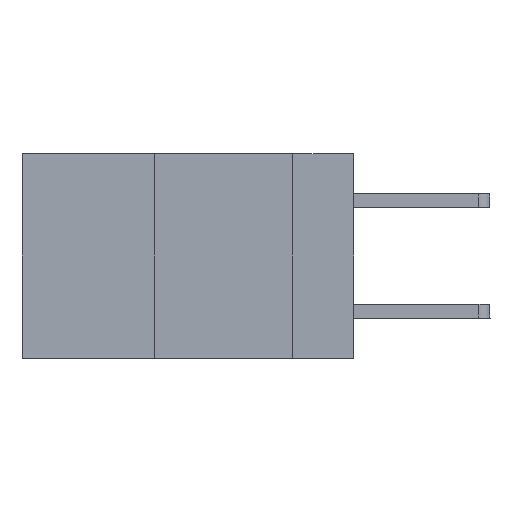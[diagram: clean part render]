
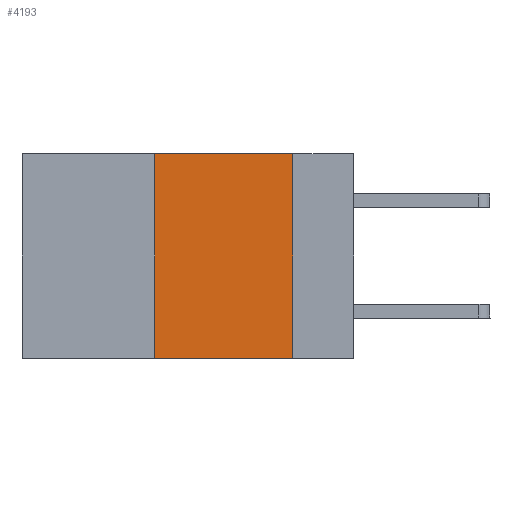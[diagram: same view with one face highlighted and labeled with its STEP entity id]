
A CAD part, left-side view. The second image highlights one B-rep face of the part: STEP entity #4193.
In plain terms, the highlighted planar face has unit normal (-1, 0, 0).
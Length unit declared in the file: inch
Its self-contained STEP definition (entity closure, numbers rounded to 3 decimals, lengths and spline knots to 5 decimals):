
#236 = DIRECTION ( 'NONE',  ( 1., 0., 0. ) ) ;
#2306 = ORIENTED_EDGE ( 'NONE', *, *, #3130, .F. ) ;
#2443 = ORIENTED_EDGE ( 'NONE', *, *, #11241, .F. ) ;
#2531 = LINE ( 'NONE', #10694, #10709 ) ;
#2547 = CARTESIAN_POINT ( 'NONE',  ( 0., 0.11, 0. ) ) ;
#2978 = VERTEX_POINT ( 'NONE', #2547 ) ;
#3130 = EDGE_CURVE ( 'NONE', #2978, #5020, #11822, .T. ) ;
#3330 = CARTESIAN_POINT ( 'NONE',  ( 0., 0.6, 0. ) ) ;
#3539 = VECTOR ( 'NONE', #10898, 39.37008 ) ;
#4193 = ADVANCED_FACE ( 'NONE', ( #6168 ), #10147, .F. ) ;
#4215 = DIRECTION ( 'NONE',  ( 0., 0., -1. ) ) ;
#4323 = CARTESIAN_POINT ( 'NONE',  ( 0., 0.11, -0.37 ) ) ;
#4570 = EDGE_CURVE ( 'NONE', #10892, #2978, #5962, .T. ) ;
#4601 = CARTESIAN_POINT ( 'NONE',  ( 0., 0.36, 0. ) ) ;
#4631 = EDGE_CURVE ( 'NONE', #7054, #5020, #2531, .T. ) ;
#4898 = LINE ( 'NONE', #12731, #5915 ) ;
#5020 = VERTEX_POINT ( 'NONE', #4323 ) ;
#5183 = CARTESIAN_POINT ( 'NONE',  ( 0., 0.6, 0. ) ) ;
#5915 = VECTOR ( 'NONE', #6897, 39.37008 ) ;
#5962 = LINE ( 'NONE', #3330, #9645 ) ;
#6168 = FACE_OUTER_BOUND ( 'NONE', #11698, .T. ) ;
#6211 = ORIENTED_EDGE ( 'NONE', *, *, #4631, .T. ) ;
#6897 = DIRECTION ( 'NONE',  ( 0., 0., 1. ) ) ;
#6903 = CARTESIAN_POINT ( 'NONE',  ( 0., 0.11, 0. ) ) ;
#7054 = VERTEX_POINT ( 'NONE', #8959 ) ;
#7273 = DIRECTION ( 'NONE',  ( 0., -1., 0. ) ) ;
#8959 = CARTESIAN_POINT ( 'NONE',  ( 0., 0.36, -0.37 ) ) ;
#9561 = DIRECTION ( 'NONE',  ( 0., -1., 0. ) ) ;
#9645 = VECTOR ( 'NONE', #7273, 39.37008 ) ;
#10147 = PLANE ( 'NONE',  #10883 ) ;
#10601 = ORIENTED_EDGE ( 'NONE', *, *, #4570, .F. ) ;
#10694 = CARTESIAN_POINT ( 'NONE',  ( 0., 0.6, -0.37 ) ) ;
#10709 = VECTOR ( 'NONE', #9561, 39.37008 ) ;
#10883 = AXIS2_PLACEMENT_3D ( 'NONE', #5183, #236, #4215 ) ;
#10892 = VERTEX_POINT ( 'NONE', #4601 ) ;
#10898 = DIRECTION ( 'NONE',  ( 0., 0., -1. ) ) ;
#11241 = EDGE_CURVE ( 'NONE', #7054, #10892, #4898, .T. ) ;
#11698 = EDGE_LOOP ( 'NONE', ( #2306, #10601, #2443, #6211 ) ) ;
#11822 = LINE ( 'NONE', #6903, #3539 ) ;
#12731 = CARTESIAN_POINT ( 'NONE',  ( 0., 0.36, 0. ) ) ;
